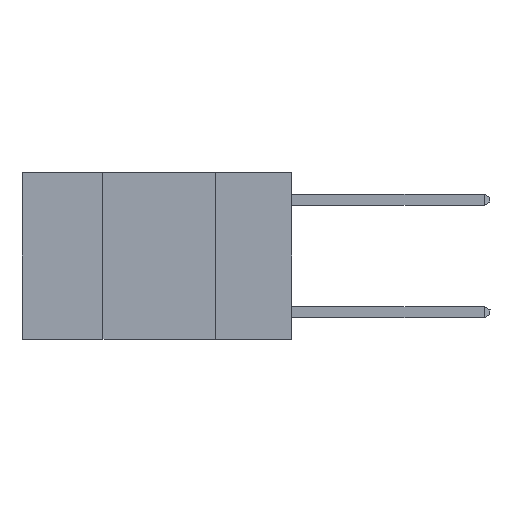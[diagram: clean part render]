
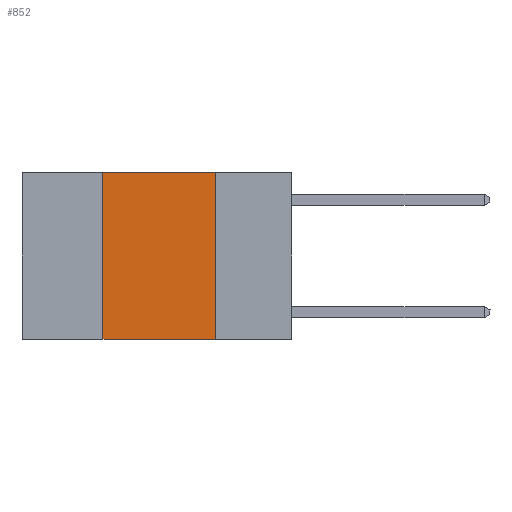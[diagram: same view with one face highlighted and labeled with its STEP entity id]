
A CAD part, left-side view. The second image highlights one B-rep face of the part: STEP entity #852.
In plain terms, the highlighted planar face has unit normal (-1, 0, 0).
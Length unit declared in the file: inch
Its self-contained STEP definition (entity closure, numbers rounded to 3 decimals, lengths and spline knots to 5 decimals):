
#2 = CARTESIAN_POINT ( 'NONE',  ( 0., 0.42, -0.37 ) ) ;
#60 = EDGE_CURVE ( 'NONE', #7571, #4167, #541, .T. ) ;
#541 = LINE ( 'NONE', #8293, #11906 ) ;
#852 = ADVANCED_FACE ( 'NONE', ( #4115 ), #8590, .F. ) ;
#1390 = EDGE_LOOP ( 'NONE', ( #3394, #9060, #3765, #6601 ) ) ;
#1855 = CARTESIAN_POINT ( 'NONE',  ( 0., 0.6, 0. ) ) ;
#1932 = CARTESIAN_POINT ( 'NONE',  ( 0., 0.17, -0.37 ) ) ;
#2261 = EDGE_CURVE ( 'NONE', #5492, #4167, #12157, .T. ) ;
#3011 = DIRECTION ( 'NONE',  ( 1., 0., 0. ) ) ;
#3394 = ORIENTED_EDGE ( 'NONE', *, *, #2261, .F. ) ;
#3504 = VECTOR ( 'NONE', #8138, 39.37008 ) ;
#3765 = ORIENTED_EDGE ( 'NONE', *, *, #11019, .F. ) ;
#4115 = FACE_OUTER_BOUND ( 'NONE', #1390, .T. ) ;
#4167 = VERTEX_POINT ( 'NONE', #1932 ) ;
#5492 = VERTEX_POINT ( 'NONE', #8868 ) ;
#5497 = VECTOR ( 'NONE', #9225, 39.37008 ) ;
#6139 = VERTEX_POINT ( 'NONE', #12998 ) ;
#6546 = DIRECTION ( 'NONE',  ( 0., 0., 1. ) ) ;
#6601 = ORIENTED_EDGE ( 'NONE', *, *, #60, .T. ) ;
#7571 = VERTEX_POINT ( 'NONE', #2 ) ;
#8138 = DIRECTION ( 'NONE',  ( 0., 0., -1. ) ) ;
#8200 = CARTESIAN_POINT ( 'NONE',  ( 0., 0.6, 0. ) ) ;
#8293 = CARTESIAN_POINT ( 'NONE',  ( 0., 0.6, -0.37 ) ) ;
#8590 = PLANE ( 'NONE',  #14015 ) ;
#8868 = CARTESIAN_POINT ( 'NONE',  ( 0., 0.17, 0. ) ) ;
#9060 = ORIENTED_EDGE ( 'NONE', *, *, #11316, .F. ) ;
#9225 = DIRECTION ( 'NONE',  ( 0., -1., 0. ) ) ;
#10686 = DIRECTION ( 'NONE',  ( 0., 0., -1. ) ) ;
#11019 = EDGE_CURVE ( 'NONE', #7571, #6139, #12047, .T. ) ;
#11316 = EDGE_CURVE ( 'NONE', #6139, #5492, #13953, .T. ) ;
#11458 = DIRECTION ( 'NONE',  ( 0., -1., 0. ) ) ;
#11906 = VECTOR ( 'NONE', #11458, 39.37008 ) ;
#12047 = LINE ( 'NONE', #12905, #12379 ) ;
#12157 = LINE ( 'NONE', #12500, #3504 ) ;
#12379 = VECTOR ( 'NONE', #6546, 39.37008 ) ;
#12500 = CARTESIAN_POINT ( 'NONE',  ( 0., 0.17, 0. ) ) ;
#12905 = CARTESIAN_POINT ( 'NONE',  ( 0., 0.42, 0. ) ) ;
#12998 = CARTESIAN_POINT ( 'NONE',  ( 0., 0.42, 0. ) ) ;
#13953 = LINE ( 'NONE', #8200, #5497 ) ;
#14015 = AXIS2_PLACEMENT_3D ( 'NONE', #1855, #3011, #10686 ) ;
